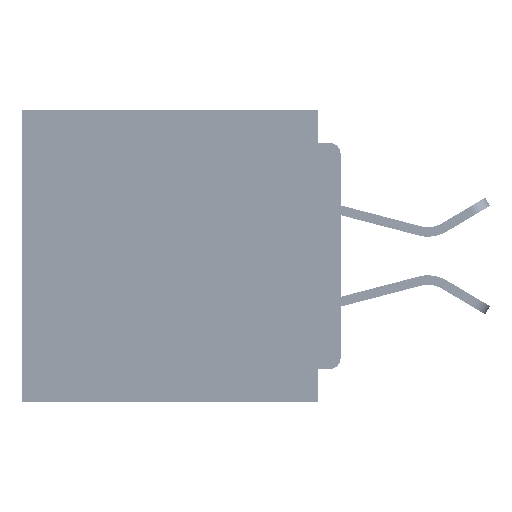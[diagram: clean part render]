
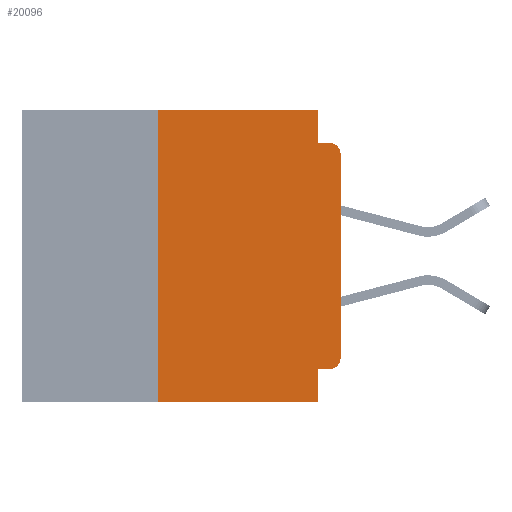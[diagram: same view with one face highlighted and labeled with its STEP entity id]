
A CAD part, left-side view. The second image highlights one B-rep face of the part: STEP entity #20096.
In plain terms, the highlighted planar face has unit normal (-1, 0, 0).
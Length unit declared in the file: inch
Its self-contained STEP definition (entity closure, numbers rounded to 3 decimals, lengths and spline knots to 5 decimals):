
#2084 = EDGE_CURVE ( 'NONE', #16763, #44562, #13861, .T. ) ;
#2936 = DIRECTION ( 'NONE',  ( 0., 0., -1. ) ) ;
#3285 = AXIS2_PLACEMENT_3D ( 'NONE', #31183, #3407, #35821 ) ;
#3407 = DIRECTION ( 'NONE',  ( -1., 0., 0. ) ) ;
#4297 = EDGE_CURVE ( 'NONE', #16763, #15209, #17286, .T. ) ;
#4767 = LINE ( 'NONE', #56037, #6240 ) ;
#4914 = DIRECTION ( 'NONE',  ( 0., 1., 0. ) ) ;
#5098 = EDGE_CURVE ( 'NONE', #6760, #15829, #55483, .T. ) ;
#5124 = CARTESIAN_POINT ( 'NONE',  ( 0., 0., -0.355 ) ) ;
#6207 = ORIENTED_EDGE ( 'NONE', *, *, #35713, .F. ) ;
#6240 = VECTOR ( 'NONE', #32866, 39.37008 ) ;
#6760 = VERTEX_POINT ( 'NONE', #39003 ) ;
#9640 = AXIS2_PLACEMENT_3D ( 'NONE', #15225, #15096, #15623 ) ;
#10632 = ORIENTED_EDGE ( 'NONE', *, *, #5098, .F. ) ;
#11392 = ORIENTED_EDGE ( 'NONE', *, *, #34816, .F. ) ;
#13016 = CARTESIAN_POINT ( 'NONE',  ( 0., 0.437, 0. ) ) ;
#13861 = CIRCLE ( 'NONE', #9640, 0.015 ) ;
#14575 = CARTESIAN_POINT ( 'NONE',  ( 0., 0., -0.06 ) ) ;
#15096 = DIRECTION ( 'NONE',  ( -1., 0., 0. ) ) ;
#15209 = VERTEX_POINT ( 'NONE', #20678 ) ;
#15225 = CARTESIAN_POINT ( 'NONE',  ( 0., 0.015, -0.34 ) ) ;
#15302 = VECTOR ( 'NONE', #26882, 39.37008 ) ;
#15623 = DIRECTION ( 'NONE',  ( 0., 0., -1. ) ) ;
#15829 = VERTEX_POINT ( 'NONE', #52475 ) ;
#15848 = VECTOR ( 'NONE', #4914, 39.37008 ) ;
#15992 = VECTOR ( 'NONE', #39643, 39.37008 ) ;
#16173 = CIRCLE ( 'NONE', #3285, 0.015 ) ;
#16537 = CARTESIAN_POINT ( 'NONE',  ( 0., 0.437, 0. ) ) ;
#16724 = LINE ( 'NONE', #13016, #50667 ) ;
#16763 = VERTEX_POINT ( 'NONE', #55821 ) ;
#16988 = CARTESIAN_POINT ( 'NONE',  ( 0., 0.015, -0.045 ) ) ;
#17105 = ORIENTED_EDGE ( 'NONE', *, *, #36800, .T. ) ;
#17167 = ORIENTED_EDGE ( 'NONE', *, *, #2084, .T. ) ;
#17222 = FACE_OUTER_BOUND ( 'NONE', #57574, .T. ) ;
#17286 = LINE ( 'NONE', #5124, #15848 ) ;
#17646 = DIRECTION ( 'NONE',  ( 0., -1., 0. ) ) ;
#18855 = DIRECTION ( 'NONE',  ( 0., 0., 1. ) ) ;
#20096 = ADVANCED_FACE ( 'NONE', ( #17222 ), #21417, .F. ) ;
#20644 = DIRECTION ( 'NONE',  ( 0., -1., 0. ) ) ;
#20678 = CARTESIAN_POINT ( 'NONE',  ( 0., 0.031, -0.355 ) ) ;
#21023 = CARTESIAN_POINT ( 'NONE',  ( 0., 0.031, -0.4 ) ) ;
#21417 = PLANE ( 'NONE',  #27019 ) ;
#21989 = CARTESIAN_POINT ( 'NONE',  ( 0., 0.25, -0.4 ) ) ;
#25411 = VERTEX_POINT ( 'NONE', #40220 ) ;
#26449 = VECTOR ( 'NONE', #20644, 39.37008 ) ;
#26882 = DIRECTION ( 'NONE',  ( 0., 0., 1. ) ) ;
#27019 = AXIS2_PLACEMENT_3D ( 'NONE', #16537, #30720, #2936 ) ;
#29208 = VERTEX_POINT ( 'NONE', #16988 ) ;
#30207 = ORIENTED_EDGE ( 'NONE', *, *, #37359, .T. ) ;
#30720 = DIRECTION ( 'NONE',  ( 1., 0., 0. ) ) ;
#30950 = VECTOR ( 'NONE', #50005, 39.37008 ) ;
#31183 = CARTESIAN_POINT ( 'NONE',  ( 0., 0.015, -0.06 ) ) ;
#32866 = DIRECTION ( 'NONE',  ( 0., 0., -1. ) ) ;
#33537 = LINE ( 'NONE', #55585, #44396 ) ;
#34594 = CARTESIAN_POINT ( 'NONE',  ( 0., 0., -0.045 ) ) ;
#34816 = EDGE_CURVE ( 'NONE', #15209, #37348, #4767, .T. ) ;
#34977 = CARTESIAN_POINT ( 'NONE',  ( 0., 0.437, -0.4 ) ) ;
#35713 = EDGE_CURVE ( 'NONE', #15829, #29208, #38771, .T. ) ;
#35821 = DIRECTION ( 'NONE',  ( 0., 0., -1. ) ) ;
#36800 = EDGE_CURVE ( 'NONE', #41689, #29208, #16173, .T. ) ;
#37348 = VERTEX_POINT ( 'NONE', #21023 ) ;
#37359 = EDGE_CURVE ( 'NONE', #50591, #37348, #40612, .T. ) ;
#38771 = LINE ( 'NONE', #34594, #26449 ) ;
#39003 = CARTESIAN_POINT ( 'NONE',  ( 0., 0.031, 0. ) ) ;
#39643 = DIRECTION ( 'NONE',  ( 0., -1., 0. ) ) ;
#39961 = LINE ( 'NONE', #45263, #15302 ) ;
#40220 = CARTESIAN_POINT ( 'NONE',  ( 0., 0.25, 0. ) ) ;
#40366 = ORIENTED_EDGE ( 'NONE', *, *, #4297, .F. ) ;
#40612 = LINE ( 'NONE', #34977, #15992 ) ;
#41032 = ORIENTED_EDGE ( 'NONE', *, *, #43283, .F. ) ;
#41618 = EDGE_CURVE ( 'NONE', #44562, #41689, #33537, .T. ) ;
#41689 = VERTEX_POINT ( 'NONE', #14575 ) ;
#43283 = EDGE_CURVE ( 'NONE', #50591, #25411, #39961, .T. ) ;
#44396 = VECTOR ( 'NONE', #18855, 39.37008 ) ;
#44441 = EDGE_CURVE ( 'NONE', #25411, #6760, #16724, .T. ) ;
#44562 = VERTEX_POINT ( 'NONE', #50535 ) ;
#45263 = CARTESIAN_POINT ( 'NONE',  ( 0., 0.25, -0.4 ) ) ;
#47481 = ORIENTED_EDGE ( 'NONE', *, *, #44441, .F. ) ;
#50005 = DIRECTION ( 'NONE',  ( 0., 0., -1. ) ) ;
#50535 = CARTESIAN_POINT ( 'NONE',  ( 0., 0., -0.34 ) ) ;
#50591 = VERTEX_POINT ( 'NONE', #21989 ) ;
#50667 = VECTOR ( 'NONE', #17646, 39.37008 ) ;
#52475 = CARTESIAN_POINT ( 'NONE',  ( 0., 0.031, -0.045 ) ) ;
#52506 = ORIENTED_EDGE ( 'NONE', *, *, #41618, .T. ) ;
#54648 = CARTESIAN_POINT ( 'NONE',  ( 0., 0.031, 0. ) ) ;
#55483 = LINE ( 'NONE', #54648, #30950 ) ;
#55585 = CARTESIAN_POINT ( 'NONE',  ( 0., 0., 0. ) ) ;
#55821 = CARTESIAN_POINT ( 'NONE',  ( 0., 0.015, -0.355 ) ) ;
#56037 = CARTESIAN_POINT ( 'NONE',  ( 0., 0.031, -0.4 ) ) ;
#57574 = EDGE_LOOP ( 'NONE', ( #52506, #17105, #6207, #10632, #47481, #41032, #30207, #11392, #40366, #17167 ) ) ;
